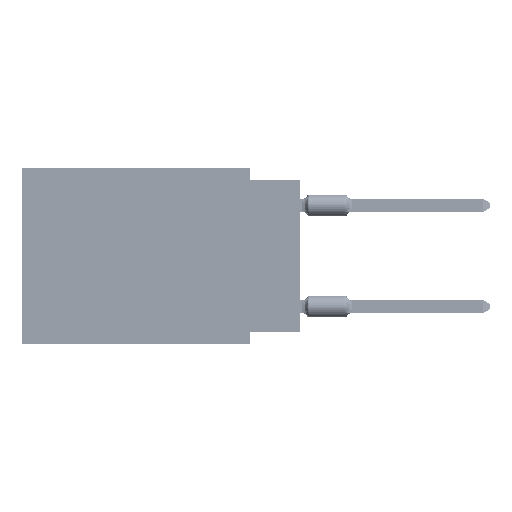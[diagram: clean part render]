
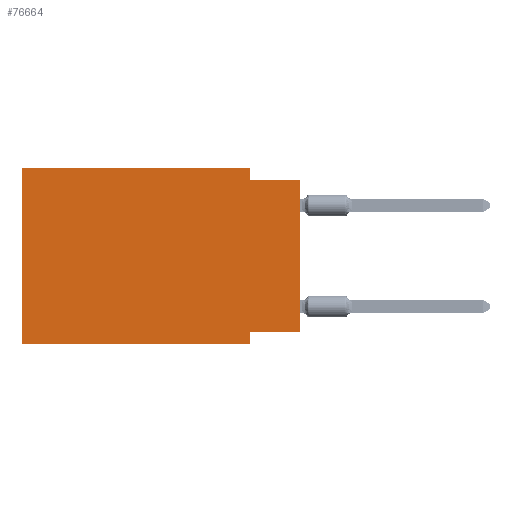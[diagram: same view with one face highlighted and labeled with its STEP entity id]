
A CAD part, left-side view. The second image highlights one B-rep face of the part: STEP entity #76664.
In plain terms, the highlighted planar face has unit normal (-1, 0, 0).
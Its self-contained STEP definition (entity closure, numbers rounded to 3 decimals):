
#547 = VERTEX_POINT ( 'NONE', #78290 ) ;
#1816 = VECTOR ( 'NONE', #56022, 1000. ) ;
#2068 = ORIENTED_EDGE ( 'NONE', *, *, #57596, .F. ) ;
#2745 = EDGE_CURVE ( 'NONE', #74870, #25175, #7812, .T. ) ;
#3929 = EDGE_CURVE ( 'NONE', #24440, #98507, #40418, .T. ) ;
#5917 = EDGE_CURVE ( 'NONE', #33052, #83226, #25728, .T. ) ;
#6615 = DIRECTION ( 'NONE',  ( 0., 0., 1. ) ) ;
#7812 = LINE ( 'NONE', #58877, #95855 ) ;
#7836 = DIRECTION ( 'NONE',  ( 1., 0., 0. ) ) ;
#7854 = LINE ( 'NONE', #26902, #31153 ) ;
#8049 = DIRECTION ( 'NONE',  ( 0., -1., 0. ) ) ;
#9032 = CARTESIAN_POINT ( 'NONE',  ( 0., 2.54, -8.255 ) ) ;
#11310 = EDGE_CURVE ( 'NONE', #24440, #33052, #7854, .T. ) ;
#16244 = PLANE ( 'NONE',  #75482 ) ;
#16900 = ORIENTED_EDGE ( 'NONE', *, *, #35898, .F. ) ;
#17934 = DIRECTION ( 'NONE',  ( 0., 1., 0. ) ) ;
#18107 = CARTESIAN_POINT ( 'NONE',  ( 0., 0., -8.255 ) ) ;
#21655 = EDGE_CURVE ( 'NONE', #50340, #83226, #23241, .T. ) ;
#21784 = CARTESIAN_POINT ( 'NONE',  ( 0., 2.54, 0. ) ) ;
#23241 = LINE ( 'NONE', #41725, #87850 ) ;
#24440 = VERTEX_POINT ( 'NONE', #18107 ) ;
#25175 = VERTEX_POINT ( 'NONE', #63654 ) ;
#25728 = LINE ( 'NONE', #44765, #66119 ) ;
#26902 = CARTESIAN_POINT ( 'NONE',  ( 0., 0., -8.255 ) ) ;
#28440 = CARTESIAN_POINT ( 'NONE',  ( 0., 0., -0.635 ) ) ;
#31153 = VECTOR ( 'NONE', #17934, 1000. ) ;
#33052 = VERTEX_POINT ( 'NONE', #9032 ) ;
#34201 = FACE_OUTER_BOUND ( 'NONE', #44154, .T. ) ;
#35802 = DIRECTION ( 'NONE',  ( 0., 0., -1. ) ) ;
#35898 = EDGE_CURVE ( 'NONE', #547, #98507, #60047, .T. ) ;
#40418 = LINE ( 'NONE', #81373, #69133 ) ;
#41725 = CARTESIAN_POINT ( 'NONE',  ( 0., 13.97, -8.89 ) ) ;
#42069 = CARTESIAN_POINT ( 'NONE',  ( 0., 13.97, 0. ) ) ;
#44154 = EDGE_LOOP ( 'NONE', ( #62767, #16900, #2068, #77555, #75739, #109103, #80231, #70288 ) ) ;
#44765 = CARTESIAN_POINT ( 'NONE',  ( 0., 2.54, -8.89 ) ) ;
#50340 = VERTEX_POINT ( 'NONE', #71078 ) ;
#50479 = CARTESIAN_POINT ( 'NONE',  ( 0., 13.97, 0. ) ) ;
#51072 = CARTESIAN_POINT ( 'NONE',  ( 0., 0., -0.635 ) ) ;
#56022 = DIRECTION ( 'NONE',  ( 0., 0., -1. ) ) ;
#57596 = EDGE_CURVE ( 'NONE', #25175, #547, #64424, .T. ) ;
#58877 = CARTESIAN_POINT ( 'NONE',  ( 0., 13.97, 0. ) ) ;
#60047 = LINE ( 'NONE', #51072, #61884 ) ;
#60593 = DIRECTION ( 'NONE',  ( 0., -1., 0. ) ) ;
#61884 = VECTOR ( 'NONE', #60593, 1000. ) ;
#62767 = ORIENTED_EDGE ( 'NONE', *, *, #3929, .T. ) ;
#63654 = CARTESIAN_POINT ( 'NONE',  ( 0., 2.54, 0. ) ) ;
#64424 = LINE ( 'NONE', #21784, #1816 ) ;
#64977 = LINE ( 'NONE', #108725, #83800 ) ;
#66119 = VECTOR ( 'NONE', #35802, 1000. ) ;
#68046 = CARTESIAN_POINT ( 'NONE',  ( 0., 2.54, -8.89 ) ) ;
#69133 = VECTOR ( 'NONE', #74644, 1000. ) ;
#70288 = ORIENTED_EDGE ( 'NONE', *, *, #11310, .F. ) ;
#71078 = CARTESIAN_POINT ( 'NONE',  ( 0., 13.97, -8.89 ) ) ;
#74644 = DIRECTION ( 'NONE',  ( 0., 0., 1. ) ) ;
#74870 = VERTEX_POINT ( 'NONE', #42069 ) ;
#75482 = AXIS2_PLACEMENT_3D ( 'NONE', #50479, #7836, #94241 ) ;
#75739 = ORIENTED_EDGE ( 'NONE', *, *, #86688, .F. ) ;
#76664 = ADVANCED_FACE ( 'NONE', ( #34201 ), #16244, .F. ) ;
#77555 = ORIENTED_EDGE ( 'NONE', *, *, #2745, .F. ) ;
#78290 = CARTESIAN_POINT ( 'NONE',  ( 0., 2.54, -0.635 ) ) ;
#80231 = ORIENTED_EDGE ( 'NONE', *, *, #5917, .F. ) ;
#81373 = CARTESIAN_POINT ( 'NONE',  ( 0., 0., 0. ) ) ;
#83226 = VERTEX_POINT ( 'NONE', #68046 ) ;
#83800 = VECTOR ( 'NONE', #6615, 1000. ) ;
#86688 = EDGE_CURVE ( 'NONE', #50340, #74870, #64977, .T. ) ;
#87850 = VECTOR ( 'NONE', #8049, 1000. ) ;
#93649 = DIRECTION ( 'NONE',  ( 0., -1., 0. ) ) ;
#94241 = DIRECTION ( 'NONE',  ( 0., 0., -1. ) ) ;
#95855 = VECTOR ( 'NONE', #93649, 1000. ) ;
#98507 = VERTEX_POINT ( 'NONE', #28440 ) ;
#108725 = CARTESIAN_POINT ( 'NONE',  ( 0., 13.97, 0. ) ) ;
#109103 = ORIENTED_EDGE ( 'NONE', *, *, #21655, .T. ) ;
